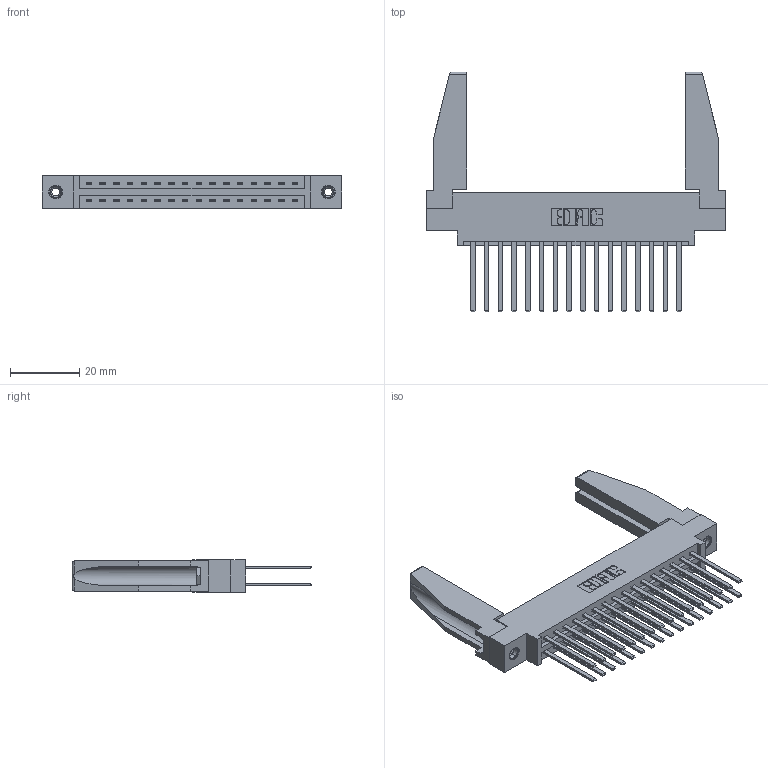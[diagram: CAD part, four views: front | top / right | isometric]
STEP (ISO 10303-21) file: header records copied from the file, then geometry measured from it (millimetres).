
FILE_DESCRIPTION (( 'STEP AP203' ), '1' );
FILE_NAME ('387-032-544-878.STEP', '2019-10-17T16:12:55', ( '' ), ( '' ), 'SwSTEP 2.0', 'SolidWorks 2016', '' );
FILE_SCHEMA (( 'CONFIG_CONTROL_DESIGN' ));
Length unit declared in the file: inch
Products named in the file (5): 337 Part_0.170 Offset - 0.156 Dia-TI; 307-220-078; 345-292-001_345-293-144; 387-032-544-878; 345-250-001_345-250-001-102
Assembly tree (37 placements, depth 2):
  387-032-544-878
    337 Part_0.170 Offset - 0.156 Dia-TI
    345-292-001_345-293-144  x32
    345-250-001_345-250-001-102  x2
    307-220-078  x2
Bounding box: 86.41 x 69.09 x 9.4 mm (x, y, z)
Volume: 13085 mm3; surface area: 15429.3 mm2
Topology: 37 solids, 37 shells, 1784 faces, 5229 edges, 3434 vertices
Faces by surface type: plane 1246, cylinder 522, cone 12, torus 4
Entity records: 18156 total; most frequent: CARTESIAN_POINT 3080, ORIENTED_EDGE 2972, DIRECTION 2670, EDGE_CURVE 1486, VECTOR 1324, LINE 1324, VERTEX_POINT 984, AXIS2_PLACEMENT_3D 673
